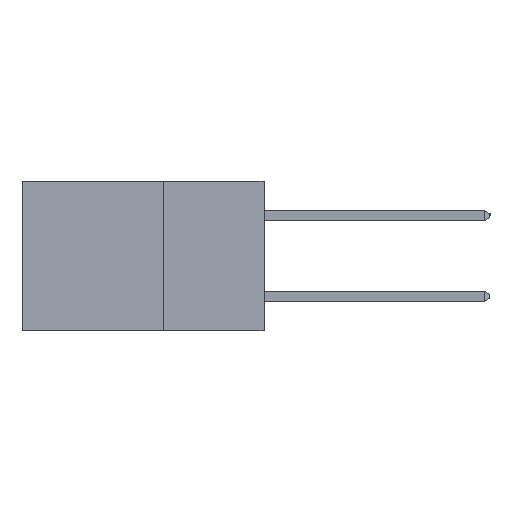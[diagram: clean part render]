
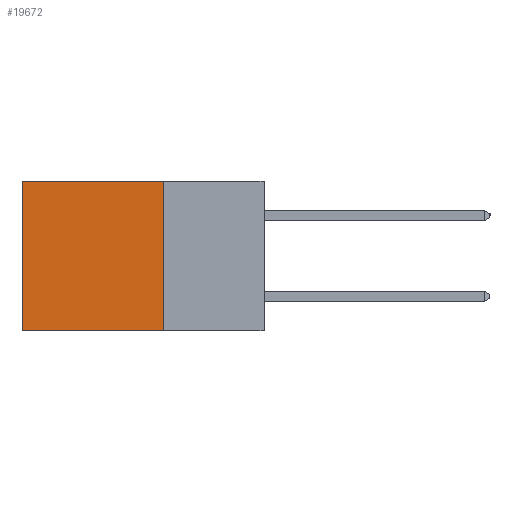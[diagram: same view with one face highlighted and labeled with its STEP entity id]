
A CAD part, left-side view. The second image highlights one B-rep face of the part: STEP entity #19672.
In plain terms, the highlighted planar face has unit normal (-1, 0, 0).
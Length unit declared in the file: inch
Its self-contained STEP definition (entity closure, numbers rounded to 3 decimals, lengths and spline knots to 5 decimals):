
#110 = ORIENTED_EDGE ( 'NONE', *, *, #8410, .T. ) ;
#908 = ORIENTED_EDGE ( 'NONE', *, *, #5785, .F. ) ;
#2024 = DIRECTION ( 'NONE',  ( 0., 0., -1. ) ) ;
#2199 = CARTESIAN_POINT ( 'NONE',  ( 0.2615, 0.25, -0.37 ) ) ;
#2755 = CARTESIAN_POINT ( 'NONE',  ( 0.2615, 0.25, -0.37 ) ) ;
#3366 = VECTOR ( 'NONE', #2024, 39.37008 ) ;
#3640 = DIRECTION ( 'NONE',  ( 0., 1., 0. ) ) ;
#4148 = PLANE ( 'NONE',  #19589 ) ;
#5233 = DIRECTION ( 'NONE',  ( 0., 1., 0. ) ) ;
#5785 = EDGE_CURVE ( 'NONE', #17878, #18042, #8254, .T. ) ;
#5845 = DIRECTION ( 'NONE',  ( 0., 0., -1. ) ) ;
#7119 = EDGE_CURVE ( 'NONE', #11173, #17878, #13417, .T. ) ;
#7385 = VERTEX_POINT ( 'NONE', #8237 ) ;
#7659 = VECTOR ( 'NONE', #5233, 39.37008 ) ;
#7755 = CARTESIAN_POINT ( 'NONE',  ( 0.2615, 0.6, -0.37 ) ) ;
#8237 = CARTESIAN_POINT ( 'NONE',  ( 0.2615, 0.6, 0. ) ) ;
#8254 = LINE ( 'NONE', #2199, #7659 ) ;
#8333 = EDGE_CURVE ( 'NONE', #11173, #7385, #11236, .T. ) ;
#8410 = EDGE_CURVE ( 'NONE', #7385, #18042, #9720, .T. ) ;
#8782 = EDGE_LOOP ( 'NONE', ( #110, #908, #9913, #19743 ) ) ;
#8888 = CARTESIAN_POINT ( 'NONE',  ( 0.2615, 0.25, -0.37 ) ) ;
#9183 = VECTOR ( 'NONE', #3640, 39.37008 ) ;
#9382 = CARTESIAN_POINT ( 'NONE',  ( 0.2615, 0.25, 0. ) ) ;
#9720 = LINE ( 'NONE', #15893, #3366 ) ;
#9913 = ORIENTED_EDGE ( 'NONE', *, *, #7119, .F. ) ;
#11173 = VERTEX_POINT ( 'NONE', #9382 ) ;
#11236 = LINE ( 'NONE', #15803, #9183 ) ;
#11915 = CARTESIAN_POINT ( 'NONE',  ( 0.2615, 0.25, -0.37 ) ) ;
#11937 = FACE_OUTER_BOUND ( 'NONE', #8782, .T. ) ;
#13417 = LINE ( 'NONE', #11915, #16076 ) ;
#13444 = DIRECTION ( 'NONE',  ( 1., 0., 0. ) ) ;
#15803 = CARTESIAN_POINT ( 'NONE',  ( 0.2615, 0.25, 0. ) ) ;
#15893 = CARTESIAN_POINT ( 'NONE',  ( 0.2615, 0.6, -0.37 ) ) ;
#16076 = VECTOR ( 'NONE', #5845, 39.37008 ) ;
#16408 = DIRECTION ( 'NONE',  ( 0., 0., -1. ) ) ;
#17878 = VERTEX_POINT ( 'NONE', #2755 ) ;
#18042 = VERTEX_POINT ( 'NONE', #7755 ) ;
#19589 = AXIS2_PLACEMENT_3D ( 'NONE', #8888, #13444, #16408 ) ;
#19672 = ADVANCED_FACE ( 'NONE', ( #11937 ), #4148, .F. ) ;
#19743 = ORIENTED_EDGE ( 'NONE', *, *, #8333, .T. ) ;
